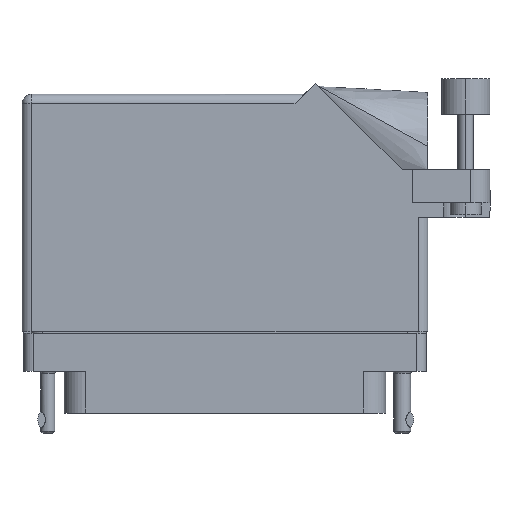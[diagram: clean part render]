
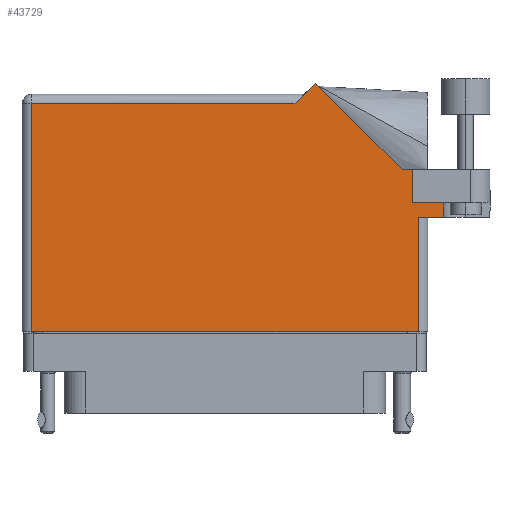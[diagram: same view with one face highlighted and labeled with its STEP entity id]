
A CAD part, front view. The second image highlights one B-rep face of the part: STEP entity #43729.
In plain terms, the highlighted face is planar.
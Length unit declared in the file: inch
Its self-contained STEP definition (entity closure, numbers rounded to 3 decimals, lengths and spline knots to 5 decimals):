
#1905 = EDGE_CURVE ( 'NONE', #45994, #54063, #49119, .T. ) ;
#2516 = CARTESIAN_POINT ( 'NONE',  ( 1.244, 0.637, 0.455 ) ) ;
#3101 = ORIENTED_EDGE ( 'NONE', *, *, #52523, .T. ) ;
#4201 = CARTESIAN_POINT ( 'NONE',  ( 1.206, 0.731, 0.455 ) ) ;
#5577 = DIRECTION ( 'NONE',  ( -1., 0., 0. ) ) ;
#5881 = PLANE ( 'NONE',  #37879 ) ;
#5968 = VECTOR ( 'NONE', #49635, 39.37008 ) ;
#6443 = DIRECTION ( 'NONE',  ( 0., -1., 0. ) ) ;
#6766 = CARTESIAN_POINT ( 'NONE',  ( -1.244, 1.368, 0.455 ) ) ;
#7175 = EDGE_LOOP ( 'NONE', ( #3101, #38222, #7369, #48381, #11055, #49239, #38123, #43436, #54372, #17841, #11749 ) ) ;
#7369 = ORIENTED_EDGE ( 'NONE', *, *, #47193, .T. ) ;
#8111 = CARTESIAN_POINT ( 'NONE',  ( 1.206, 0.944, 0.455 ) ) ;
#8140 = VERTEX_POINT ( 'NONE', #8111 ) ;
#8283 = VERTEX_POINT ( 'NONE', #51944 ) ;
#8843 = EDGE_CURVE ( 'NONE', #37414, #45408, #58061, .T. ) ;
#10236 = DIRECTION ( 'NONE',  ( 0., 0., -1. ) ) ;
#11034 = CARTESIAN_POINT ( 'NONE',  ( 1.14042, 0.944, 0.455 ) ) ;
#11055 = ORIENTED_EDGE ( 'NONE', *, *, #58583, .F. ) ;
#11259 = LINE ( 'NONE', #44536, #31247 ) ;
#11749 = ORIENTED_EDGE ( 'NONE', *, *, #33080, .T. ) ;
#12763 = LINE ( 'NONE', #2516, #61188 ) ;
#13104 = LINE ( 'NONE', #40800, #42522 ) ;
#13132 = LINE ( 'NONE', #45789, #57338 ) ;
#13580 = CARTESIAN_POINT ( 'NONE',  ( 0.58371, 1.50071, 0.455 ) ) ;
#14477 = CARTESIAN_POINT ( 'NONE',  ( 1.306, 0.637, 0.455 ) ) ;
#14855 = LINE ( 'NONE', #23571, #21732 ) ;
#17841 = ORIENTED_EDGE ( 'NONE', *, *, #1905, .T. ) ;
#18520 = VERTEX_POINT ( 'NONE', #29348 ) ;
#21193 = DIRECTION ( 'NONE',  ( 0., 1., 0. ) ) ;
#21732 = VECTOR ( 'NONE', #60889, 39.37008 ) ;
#23571 = CARTESIAN_POINT ( 'NONE',  ( -1.306, -0.1, 0.455 ) ) ;
#24106 = LINE ( 'NONE', #14477, #49991 ) ;
#24577 = CARTESIAN_POINT ( 'NONE',  ( -1.306, 1.368, 0.455 ) ) ;
#25324 = CARTESIAN_POINT ( 'NONE',  ( 1.706, 0.944, 0.455 ) ) ;
#28969 = EDGE_CURVE ( 'NONE', #18520, #8283, #12763, .T. ) ;
#29348 = CARTESIAN_POINT ( 'NONE',  ( 1.244, -0.1, 0.455 ) ) ;
#30085 = VERTEX_POINT ( 'NONE', #4201 ) ;
#31247 = VECTOR ( 'NONE', #58838, 39.37008 ) ;
#33080 = EDGE_CURVE ( 'NONE', #54063, #35675, #45272, .T. ) ;
#33887 = FACE_OUTER_BOUND ( 'NONE', #7175, .T. ) ;
#34497 = LINE ( 'NONE', #36617, #44905 ) ;
#34657 = DIRECTION ( 'NONE',  ( -1., 0., 0. ) ) ;
#34748 = EDGE_CURVE ( 'NONE', #8140, #55840, #43676, .T. ) ;
#35675 = VERTEX_POINT ( 'NONE', #42918 ) ;
#36617 = CARTESIAN_POINT ( 'NONE',  ( 1.14042, 0.944, 0.455 ) ) ;
#37414 = VERTEX_POINT ( 'NONE', #44355 ) ;
#37879 = AXIS2_PLACEMENT_3D ( 'NONE', #52841, #10236, #5577 ) ;
#38123 = ORIENTED_EDGE ( 'NONE', *, *, #34748, .T. ) ;
#38222 = ORIENTED_EDGE ( 'NONE', *, *, #28969, .T. ) ;
#39803 = DIRECTION ( 'NONE',  ( -1., 0., 0. ) ) ;
#40800 = CARTESIAN_POINT ( 'NONE',  ( 1.206, 0.731, 0.455 ) ) ;
#40850 = VERTEX_POINT ( 'NONE', #13580 ) ;
#42522 = VECTOR ( 'NONE', #59160, 39.37008 ) ;
#42918 = CARTESIAN_POINT ( 'NONE',  ( -1.244, -0.1, 0.455 ) ) ;
#43436 = ORIENTED_EDGE ( 'NONE', *, *, #43867, .T. ) ;
#43676 = LINE ( 'NONE', #25324, #48618 ) ;
#43729 = ADVANCED_FACE ( 'NONE', ( #33887 ), #5881, .F. ) ;
#43867 = EDGE_CURVE ( 'NONE', #55840, #40850, #34497, .T. ) ;
#44355 = CARTESIAN_POINT ( 'NONE',  ( 1.4075, 0.731, 0.455 ) ) ;
#44536 = CARTESIAN_POINT ( 'NONE',  ( 0.513, 1.43, 0.455 ) ) ;
#44905 = VECTOR ( 'NONE', #45946, 39.37008 ) ;
#45272 = LINE ( 'NONE', #54611, #5968 ) ;
#45408 = VERTEX_POINT ( 'NONE', #47184 ) ;
#45789 = CARTESIAN_POINT ( 'NONE',  ( 1.206, 0.731, 0.455 ) ) ;
#45946 = DIRECTION ( 'NONE',  ( -0.707, 0.707, 0. ) ) ;
#45994 = VERTEX_POINT ( 'NONE', #57664 ) ;
#47184 = CARTESIAN_POINT ( 'NONE',  ( 1.4075, 0.637, 0.455 ) ) ;
#47193 = EDGE_CURVE ( 'NONE', #8283, #45408, #24106, .T. ) ;
#48381 = ORIENTED_EDGE ( 'NONE', *, *, #8843, .F. ) ;
#48618 = VECTOR ( 'NONE', #34657, 39.37008 ) ;
#49119 = LINE ( 'NONE', #24577, #60512 ) ;
#49239 = ORIENTED_EDGE ( 'NONE', *, *, #58114, .T. ) ;
#49635 = DIRECTION ( 'NONE',  ( 0., -1., 0. ) ) ;
#49991 = VECTOR ( 'NONE', #57985, 39.37008 ) ;
#51944 = CARTESIAN_POINT ( 'NONE',  ( 1.244, 0.637, 0.455 ) ) ;
#52523 = EDGE_CURVE ( 'NONE', #35675, #18520, #14855, .T. ) ;
#52841 = CARTESIAN_POINT ( 'NONE',  ( -1.306, 1.43, 0.455 ) ) ;
#53401 = CARTESIAN_POINT ( 'NONE',  ( 1.4075, 1.06177, 0.455 ) ) ;
#54063 = VERTEX_POINT ( 'NONE', #6766 ) ;
#54372 = ORIENTED_EDGE ( 'NONE', *, *, #54946, .T. ) ;
#54611 = CARTESIAN_POINT ( 'NONE',  ( -1.244, -0.1, 0.455 ) ) ;
#54946 = EDGE_CURVE ( 'NONE', #40850, #45994, #11259, .T. ) ;
#55431 = DIRECTION ( 'NONE',  ( 0., 1., 0. ) ) ;
#55840 = VERTEX_POINT ( 'NONE', #11034 ) ;
#57338 = VECTOR ( 'NONE', #55431, 39.37008 ) ;
#57664 = CARTESIAN_POINT ( 'NONE',  ( 0.451, 1.368, 0.455 ) ) ;
#57985 = DIRECTION ( 'NONE',  ( 1., 0., 0. ) ) ;
#58061 = LINE ( 'NONE', #53401, #58167 ) ;
#58114 = EDGE_CURVE ( 'NONE', #30085, #8140, #13132, .T. ) ;
#58167 = VECTOR ( 'NONE', #6443, 39.37008 ) ;
#58583 = EDGE_CURVE ( 'NONE', #30085, #37414, #13104, .T. ) ;
#58838 = DIRECTION ( 'NONE',  ( -0.707, -0.707, 0. ) ) ;
#59160 = DIRECTION ( 'NONE',  ( 1., 0., 0. ) ) ;
#60512 = VECTOR ( 'NONE', #39803, 39.37008 ) ;
#60889 = DIRECTION ( 'NONE',  ( 1., 0., 0. ) ) ;
#61188 = VECTOR ( 'NONE', #21193, 39.37008 ) ;
